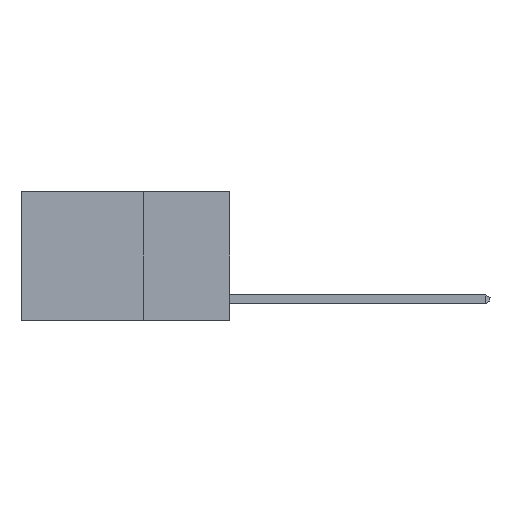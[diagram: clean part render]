
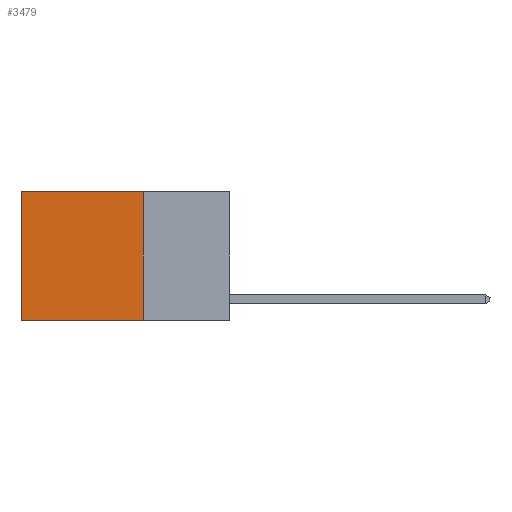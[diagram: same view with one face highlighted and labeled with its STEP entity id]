
A CAD part, left-side view. The second image highlights one B-rep face of the part: STEP entity #3479.
In plain terms, the highlighted planar face has unit normal (-1, 0, 0).
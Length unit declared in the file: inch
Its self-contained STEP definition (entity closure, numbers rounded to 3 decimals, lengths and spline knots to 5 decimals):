
#1251 = ORIENTED_EDGE ( 'NONE', *, *, #2910, .F. ) ;
#1502 = LINE ( 'NONE', #8677, #10410 ) ;
#1946 = EDGE_LOOP ( 'NONE', ( #4672, #1251, #5585, #9981 ) ) ;
#1955 = CARTESIAN_POINT ( 'NONE',  ( 0.2625, 0.25, 0. ) ) ;
#2054 = VECTOR ( 'NONE', #12720, 39.37008 ) ;
#2375 = VERTEX_POINT ( 'NONE', #4196 ) ;
#2425 = VECTOR ( 'NONE', #10086, 39.37008 ) ;
#2910 = EDGE_CURVE ( 'NONE', #5067, #13021, #5138, .T. ) ;
#3479 = ADVANCED_FACE ( 'NONE', ( #9639 ), #10199, .F. ) ;
#3520 = CARTESIAN_POINT ( 'NONE',  ( 0.2625, 0.25, 0. ) ) ;
#4107 = AXIS2_PLACEMENT_3D ( 'NONE', #6800, #14696, #7951 ) ;
#4196 = CARTESIAN_POINT ( 'NONE',  ( 0.2625, 0.25, 0. ) ) ;
#4672 = ORIENTED_EDGE ( 'NONE', *, *, #8819, .T. ) ;
#5067 = VERTEX_POINT ( 'NONE', #8583 ) ;
#5132 = CARTESIAN_POINT ( 'NONE',  ( 0.2625, 0.25, -0.37 ) ) ;
#5138 = LINE ( 'NONE', #5132, #8224 ) ;
#5189 = DIRECTION ( 'NONE',  ( 0., 1., 0. ) ) ;
#5480 = CARTESIAN_POINT ( 'NONE',  ( 0.2625, 0.6, 0. ) ) ;
#5585 = ORIENTED_EDGE ( 'NONE', *, *, #8502, .F. ) ;
#6800 = CARTESIAN_POINT ( 'NONE',  ( 0.2625, 0.25, 0. ) ) ;
#7244 = CARTESIAN_POINT ( 'NONE',  ( 0.2625, 0.6, -0.37 ) ) ;
#7951 = DIRECTION ( 'NONE',  ( 0., 0., -1. ) ) ;
#8224 = VECTOR ( 'NONE', #5189, 39.37008 ) ;
#8279 = LINE ( 'NONE', #3520, #2054 ) ;
#8502 = EDGE_CURVE ( 'NONE', #2375, #5067, #8279, .T. ) ;
#8583 = CARTESIAN_POINT ( 'NONE',  ( 0.2625, 0.25, -0.37 ) ) ;
#8677 = CARTESIAN_POINT ( 'NONE',  ( 0.2625, 0.6, 0. ) ) ;
#8819 = EDGE_CURVE ( 'NONE', #12739, #13021, #1502, .T. ) ;
#9639 = FACE_OUTER_BOUND ( 'NONE', #1946, .T. ) ;
#9981 = ORIENTED_EDGE ( 'NONE', *, *, #13327, .T. ) ;
#10086 = DIRECTION ( 'NONE',  ( 0., 1., 0. ) ) ;
#10199 = PLANE ( 'NONE',  #4107 ) ;
#10410 = VECTOR ( 'NONE', #12084, 39.37008 ) ;
#12084 = DIRECTION ( 'NONE',  ( 0., 0., -1. ) ) ;
#12720 = DIRECTION ( 'NONE',  ( 0., 0., -1. ) ) ;
#12739 = VERTEX_POINT ( 'NONE', #5480 ) ;
#13021 = VERTEX_POINT ( 'NONE', #7244 ) ;
#13327 = EDGE_CURVE ( 'NONE', #2375, #12739, #13894, .T. ) ;
#13894 = LINE ( 'NONE', #1955, #2425 ) ;
#14696 = DIRECTION ( 'NONE',  ( 1., 0., 0. ) ) ;
